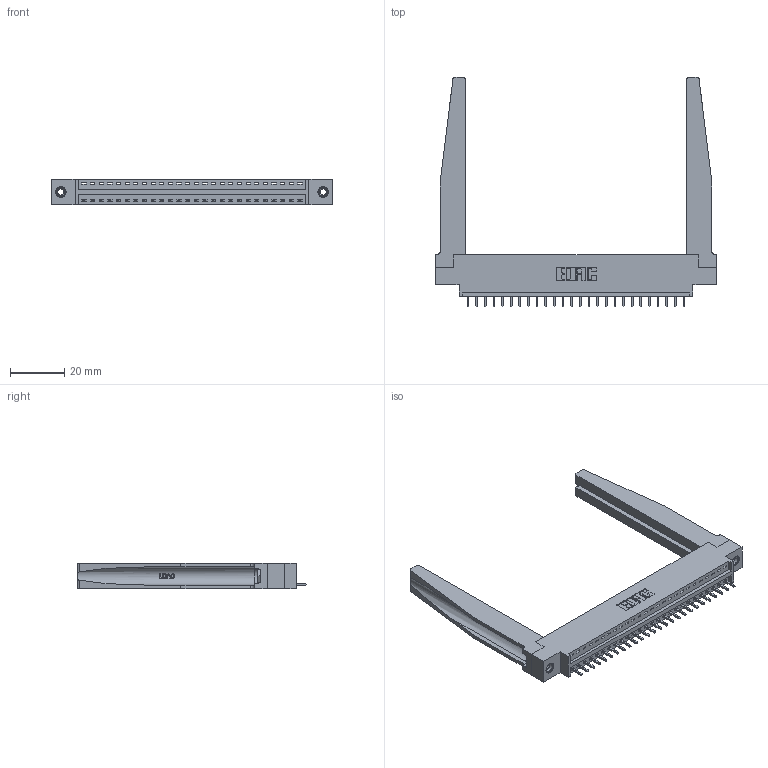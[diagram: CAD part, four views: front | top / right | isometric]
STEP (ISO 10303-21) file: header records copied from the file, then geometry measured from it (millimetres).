
FILE_DESCRIPTION (( 'STEP AP203' ), '1' );
FILE_NAME ('396-026-521-678.STEP', '2019-10-27T07:05:58', ( '' ), ( '' ), 'SwSTEP 2.0', 'SolidWorks 2016', '' );
FILE_SCHEMA (( 'CONFIG_CONTROL_DESIGN' ));
Length unit declared in the file: inch
Products named in the file (5): 396-026-521-678; 345-292-001_345-293-121; 346-220-078_345-220-078; 346 Part_0.170 Offset - 0.156 Dia-TH; 345-250-001_345-250-001-102
Assembly tree (31 placements, depth 2):
  396-026-521-678
    346 Part_0.170 Offset - 0.156 Dia-TH
    345-292-001_345-293-121  x26
    346-220-078_345-220-078  x2
    345-250-001_345-250-001-102  x2
Bounding box: 103.12 x 84.33 x 9.4 mm (x, y, z)
Volume: 16441.3 mm3; surface area: 18147.8 mm2
Topology: 31 solids, 31 shells, 1868 faces, 5525 edges, 3638 vertices
Faces by surface type: plane 1262, cylinder 554, bspline 36, cone 12, torus 4
Entity records: 23188 total; most frequent: CARTESIAN_POINT 4893, ORIENTED_EDGE 3742, DIRECTION 3321, EDGE_CURVE 1871, LINE 1541, VECTOR 1541, VERTEX_POINT 1240, AXIS2_PLACEMENT_3D 890
